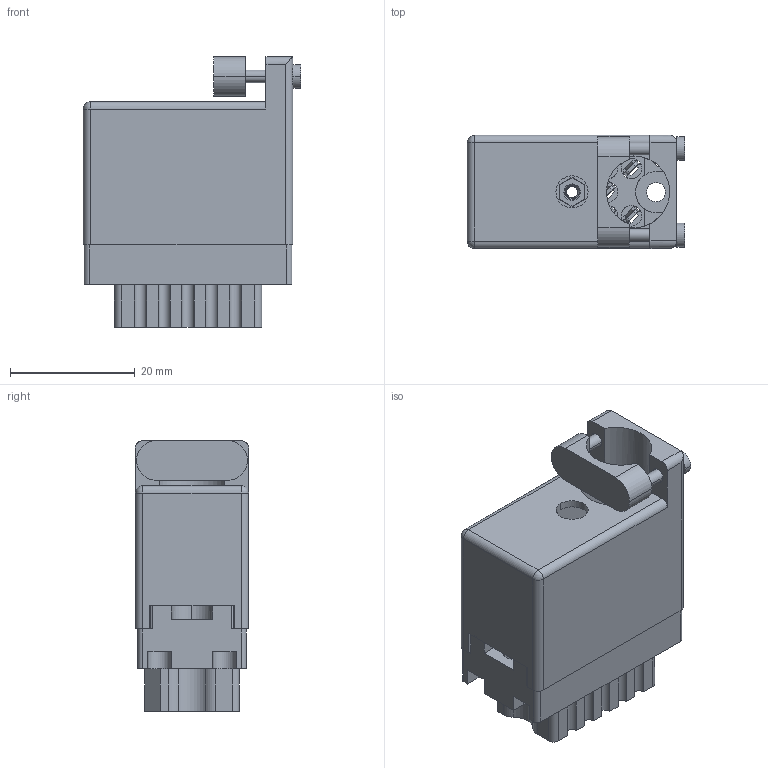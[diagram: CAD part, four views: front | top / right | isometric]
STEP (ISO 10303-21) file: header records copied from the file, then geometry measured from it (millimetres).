
FILE_DESCRIPTION (( 'STEP AP203' ), '1' );
FILE_NAME ('519-014-501-416.STEP', '2020-09-09T18:26:19', ( '' ), ( '' ), 'SwSTEP 2.0', 'SolidWorks 2020', '' );
FILE_SCHEMA (( 'CONFIG_CONTROL_DESIGN' ));
Length unit declared in the file: inch
Products named in the file (5): 516-292-001_501 Contact; 519 Receptacle Insulator_014; 516-252-025-100_516-252-025-100; 516-230-001_Plastic - 020 Top Entry; 519-014-501-416
Assembly tree (17 placements, depth 2):
  519-014-501-416
    519 Receptacle Insulator_014
    516-292-001_501 Contact  x14
    516-252-025-100_516-252-025-100
    516-230-001_Plastic - 020 Top Entry
Bounding box: 34.92 x 18.16 x 43.46 mm (x, y, z)
Volume: 10506.9 mm3; surface area: 15833.8 mm2
Topology: 17 solids, 17 shells, 1603 faces, 4627 edges, 3065 vertices
Faces by surface type: plane 937, cylinder 566, bspline 87, cone 11, sphere 2
Entity records: 25675 total; most frequent: CARTESIAN_POINT 6906, ORIENTED_EDGE 3842, DIRECTION 3682, EDGE_CURVE 1921, VECTOR 1324, LINE 1324, VERTEX_POINT 1271, AXIS2_PLACEMENT_3D 1179
